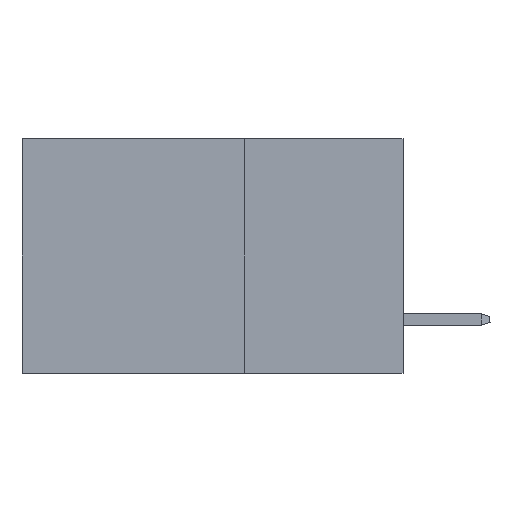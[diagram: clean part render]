
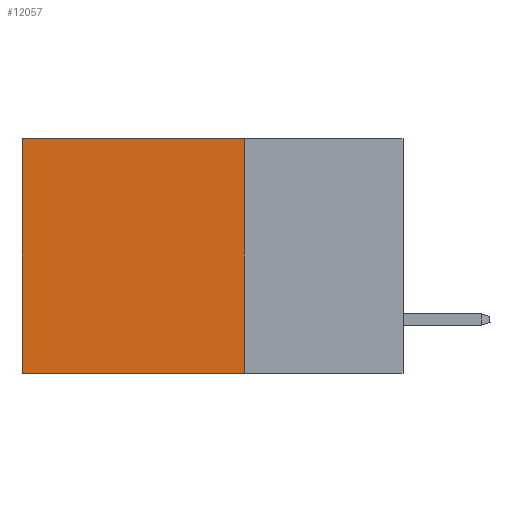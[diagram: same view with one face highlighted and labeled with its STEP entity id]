
A CAD part, left-side view. The second image highlights one B-rep face of the part: STEP entity #12057.
In plain terms, the highlighted planar face has unit normal (-1, 0, 0).
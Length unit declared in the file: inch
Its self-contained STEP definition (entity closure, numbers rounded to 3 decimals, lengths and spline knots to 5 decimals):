
#686 = LINE ( 'NONE', #18286, #10788 ) ;
#730 = LINE ( 'NONE', #9723, #2792 ) ;
#815 = CARTESIAN_POINT ( 'NONE',  ( 0.2875, 0.6, -0.37 ) ) ;
#2627 = DIRECTION ( 'NONE',  ( 0., 1., 0. ) ) ;
#2792 = VECTOR ( 'NONE', #8008, 39.37008 ) ;
#3574 = LINE ( 'NONE', #21706, #8659 ) ;
#3779 = EDGE_CURVE ( 'NONE', #11075, #16769, #686, .T. ) ;
#4488 = CARTESIAN_POINT ( 'NONE',  ( 0.2875, 0.25, -0.37 ) ) ;
#4494 = FACE_OUTER_BOUND ( 'NONE', #18691, .T. ) ;
#4815 = VERTEX_POINT ( 'NONE', #4488 ) ;
#6330 = PLANE ( 'NONE',  #8900 ) ;
#6782 = ORIENTED_EDGE ( 'NONE', *, *, #7809, .F. ) ;
#6855 = CARTESIAN_POINT ( 'NONE',  ( 0.2875, 0.25, 0. ) ) ;
#7489 = VECTOR ( 'NONE', #20222, 39.37008 ) ;
#7809 = EDGE_CURVE ( 'NONE', #21783, #4815, #730, .T. ) ;
#8008 = DIRECTION ( 'NONE',  ( 0., 0., -1. ) ) ;
#8049 = ORIENTED_EDGE ( 'NONE', *, *, #3779, .T. ) ;
#8659 = VECTOR ( 'NONE', #2627, 39.37008 ) ;
#8900 = AXIS2_PLACEMENT_3D ( 'NONE', #9625, #20371, #13086 ) ;
#9625 = CARTESIAN_POINT ( 'NONE',  ( 0.2875, 0.25, 0. ) ) ;
#9723 = CARTESIAN_POINT ( 'NONE',  ( 0.2875, 0.25, 0. ) ) ;
#10788 = VECTOR ( 'NONE', #11090, 39.37008 ) ;
#11075 = VERTEX_POINT ( 'NONE', #13587 ) ;
#11090 = DIRECTION ( 'NONE',  ( 0., 0., -1. ) ) ;
#11791 = CARTESIAN_POINT ( 'NONE',  ( 0.2875, 0.25, 0. ) ) ;
#12057 = ADVANCED_FACE ( 'NONE', ( #4494 ), #6330, .F. ) ;
#13086 = DIRECTION ( 'NONE',  ( 0., 0., -1. ) ) ;
#13173 = EDGE_CURVE ( 'NONE', #21783, #11075, #13373, .T. ) ;
#13373 = LINE ( 'NONE', #11791, #7489 ) ;
#13587 = CARTESIAN_POINT ( 'NONE',  ( 0.2875, 0.6, 0. ) ) ;
#16769 = VERTEX_POINT ( 'NONE', #815 ) ;
#17141 = EDGE_CURVE ( 'NONE', #4815, #16769, #3574, .T. ) ;
#17732 = ORIENTED_EDGE ( 'NONE', *, *, #17141, .F. ) ;
#18286 = CARTESIAN_POINT ( 'NONE',  ( 0.2875, 0.6, 0. ) ) ;
#18691 = EDGE_LOOP ( 'NONE', ( #8049, #17732, #6782, #20318 ) ) ;
#20222 = DIRECTION ( 'NONE',  ( 0., 1., 0. ) ) ;
#20318 = ORIENTED_EDGE ( 'NONE', *, *, #13173, .T. ) ;
#20371 = DIRECTION ( 'NONE',  ( 1., 0., 0. ) ) ;
#21706 = CARTESIAN_POINT ( 'NONE',  ( 0.2875, 0.25, -0.37 ) ) ;
#21783 = VERTEX_POINT ( 'NONE', #6855 ) ;
